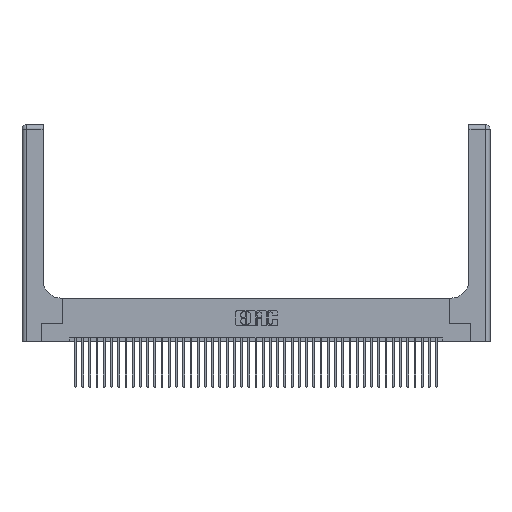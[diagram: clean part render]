
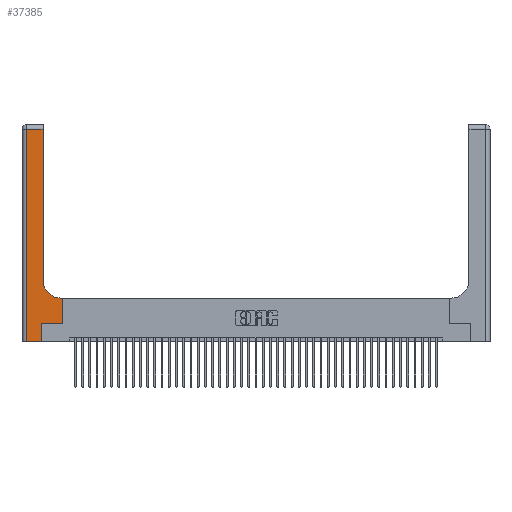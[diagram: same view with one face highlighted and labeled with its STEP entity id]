
A CAD part, top view. The second image highlights one B-rep face of the part: STEP entity #37385.
In plain terms, the highlighted planar face has unit normal (0, 0, 1).
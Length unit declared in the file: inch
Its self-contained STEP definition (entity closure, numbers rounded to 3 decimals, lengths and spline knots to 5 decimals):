
#770 = VECTOR ( 'NONE', #40119, 39.37008 ) ;
#908 = ORIENTED_EDGE ( 'NONE', *, *, #32151, .T. ) ;
#959 = VERTEX_POINT ( 'NONE', #17430 ) ;
#1682 = VERTEX_POINT ( 'NONE', #35191 ) ;
#2202 = VERTEX_POINT ( 'NONE', #37357 ) ;
#2557 = VERTEX_POINT ( 'NONE', #20447 ) ;
#2629 = AXIS2_PLACEMENT_3D ( 'NONE', #32517, #8233, #18276 ) ;
#2694 = CARTESIAN_POINT ( 'NONE',  ( 0.06, 3., 0.37 ) ) ;
#3233 = DIRECTION ( 'NONE',  ( 0., 0., -1. ) ) ;
#3404 = VERTEX_POINT ( 'NONE', #21627 ) ;
#5699 = ORIENTED_EDGE ( 'NONE', *, *, #27949, .T. ) ;
#6185 = ORIENTED_EDGE ( 'NONE', *, *, #22118, .T. ) ;
#6194 = CARTESIAN_POINT ( 'NONE',  ( 0.5585, 0.25, 0.37 ) ) ;
#6591 = CARTESIAN_POINT ( 'NONE',  ( 0.269, 0.25, 0.37 ) ) ;
#6642 = LINE ( 'NONE', #34727, #42871 ) ;
#7741 = ORIENTED_EDGE ( 'NONE', *, *, #13256, .T. ) ;
#8233 = DIRECTION ( 'NONE',  ( 0., 0., -1. ) ) ;
#9970 = VERTEX_POINT ( 'NONE', #6591 ) ;
#10536 = EDGE_CURVE ( 'NONE', #959, #1682, #34504, .T. ) ;
#12667 = EDGE_CURVE ( 'NONE', #3404, #23829, #28427, .T. ) ;
#13232 = VERTEX_POINT ( 'NONE', #32163 ) ;
#13256 = EDGE_CURVE ( 'NONE', #2557, #959, #31679, .T. ) ;
#13404 = ORIENTED_EDGE ( 'NONE', *, *, #17910, .T. ) ;
#14596 = VECTOR ( 'NONE', #24155, 39.37008 ) ;
#16302 = DIRECTION ( 'NONE',  ( 0., 1., 0. ) ) ;
#16758 = EDGE_CURVE ( 'NONE', #1682, #3404, #17447, .T. ) ;
#16867 = PLANE ( 'NONE',  #20686 ) ;
#16953 = VECTOR ( 'NONE', #30074, 39.37008 ) ;
#17208 = CARTESIAN_POINT ( 'NONE',  ( 0.269, 0., 0.37 ) ) ;
#17430 = CARTESIAN_POINT ( 'NONE',  ( 0.2915, 2.94, 0.37 ) ) ;
#17447 = LINE ( 'NONE', #2694, #16953 ) ;
#17612 = FACE_OUTER_BOUND ( 'NONE', #25397, .T. ) ;
#17910 = EDGE_CURVE ( 'NONE', #18354, #13232, #6642, .T. ) ;
#18276 = DIRECTION ( 'NONE',  ( 1., 0., 0. ) ) ;
#18354 = VERTEX_POINT ( 'NONE', #39303 ) ;
#19922 = DIRECTION ( 'NONE',  ( 0., 1., 0. ) ) ;
#20093 = CARTESIAN_POINT ( 'NONE',  ( 0., 0., 0.37 ) ) ;
#20447 = CARTESIAN_POINT ( 'NONE',  ( 0.2915, 0.85, 0.37 ) ) ;
#20686 = AXIS2_PLACEMENT_3D ( 'NONE', #40594, #3233, #23696 ) ;
#21627 = CARTESIAN_POINT ( 'NONE',  ( 0.06, 0., 0.37 ) ) ;
#22118 = EDGE_CURVE ( 'NONE', #2202, #18354, #33417, .T. ) ;
#22984 = CARTESIAN_POINT ( 'NONE',  ( 0.2915, 3., 0.37 ) ) ;
#23696 = DIRECTION ( 'NONE',  ( -1., 0., 0. ) ) ;
#23829 = VERTEX_POINT ( 'NONE', #17208 ) ;
#24155 = DIRECTION ( 'NONE',  ( 1., 0., 0. ) ) ;
#24830 = DIRECTION ( 'NONE',  ( 0., 1., 0. ) ) ;
#25397 = EDGE_LOOP ( 'NONE', ( #7741, #35905, #43021, #33787, #908, #5699, #6185, #13404, #41789 ) ) ;
#27949 = EDGE_CURVE ( 'NONE', #9970, #2202, #32109, .T. ) ;
#28427 = LINE ( 'NONE', #20093, #770 ) ;
#29440 = EDGE_CURVE ( 'NONE', #13232, #2557, #31984, .T. ) ;
#30074 = DIRECTION ( 'NONE',  ( 0., -1., 0. ) ) ;
#30597 = VECTOR ( 'NONE', #16302, 39.37008 ) ;
#30648 = CARTESIAN_POINT ( 'NONE',  ( 0., 2.94, 0.37 ) ) ;
#31679 = LINE ( 'NONE', #22984, #30597 ) ;
#31984 = CIRCLE ( 'NONE', #2629, 0.25 ) ;
#32109 = LINE ( 'NONE', #41053, #14596 ) ;
#32151 = EDGE_CURVE ( 'NONE', #23829, #9970, #44014, .T. ) ;
#32163 = CARTESIAN_POINT ( 'NONE',  ( 0.5415, 0.6, 0.37 ) ) ;
#32517 = CARTESIAN_POINT ( 'NONE',  ( 0.5415, 0.85, 0.37 ) ) ;
#33417 = LINE ( 'NONE', #6194, #39761 ) ;
#33787 = ORIENTED_EDGE ( 'NONE', *, *, #12667, .T. ) ;
#34077 = DIRECTION ( 'NONE',  ( -1., 0., 0. ) ) ;
#34438 = VECTOR ( 'NONE', #24830, 39.37008 ) ;
#34504 = LINE ( 'NONE', #30648, #37689 ) ;
#34727 = CARTESIAN_POINT ( 'NONE',  ( 0.2915, 0.6, 0.37 ) ) ;
#34749 = CARTESIAN_POINT ( 'NONE',  ( 0.269, 0., 0.37 ) ) ;
#35191 = CARTESIAN_POINT ( 'NONE',  ( 0.06, 2.94, 0.37 ) ) ;
#35905 = ORIENTED_EDGE ( 'NONE', *, *, #10536, .T. ) ;
#37357 = CARTESIAN_POINT ( 'NONE',  ( 0.5585, 0.25, 0.37 ) ) ;
#37385 = ADVANCED_FACE ( 'NONE', ( #17612 ), #16867, .F. ) ;
#37689 = VECTOR ( 'NONE', #34077, 39.37008 ) ;
#39303 = CARTESIAN_POINT ( 'NONE',  ( 0.5585, 0.6, 0.37 ) ) ;
#39761 = VECTOR ( 'NONE', #19922, 39.37008 ) ;
#40119 = DIRECTION ( 'NONE',  ( 1., 0., 0. ) ) ;
#40594 = CARTESIAN_POINT ( 'NONE',  ( 0., 3., 0.37 ) ) ;
#41053 = CARTESIAN_POINT ( 'NONE',  ( 0.269, 0.25, 0.37 ) ) ;
#41789 = ORIENTED_EDGE ( 'NONE', *, *, #29440, .T. ) ;
#42161 = DIRECTION ( 'NONE',  ( -1., 0., 0. ) ) ;
#42871 = VECTOR ( 'NONE', #42161, 39.37008 ) ;
#43021 = ORIENTED_EDGE ( 'NONE', *, *, #16758, .T. ) ;
#44014 = LINE ( 'NONE', #34749, #34438 ) ;
